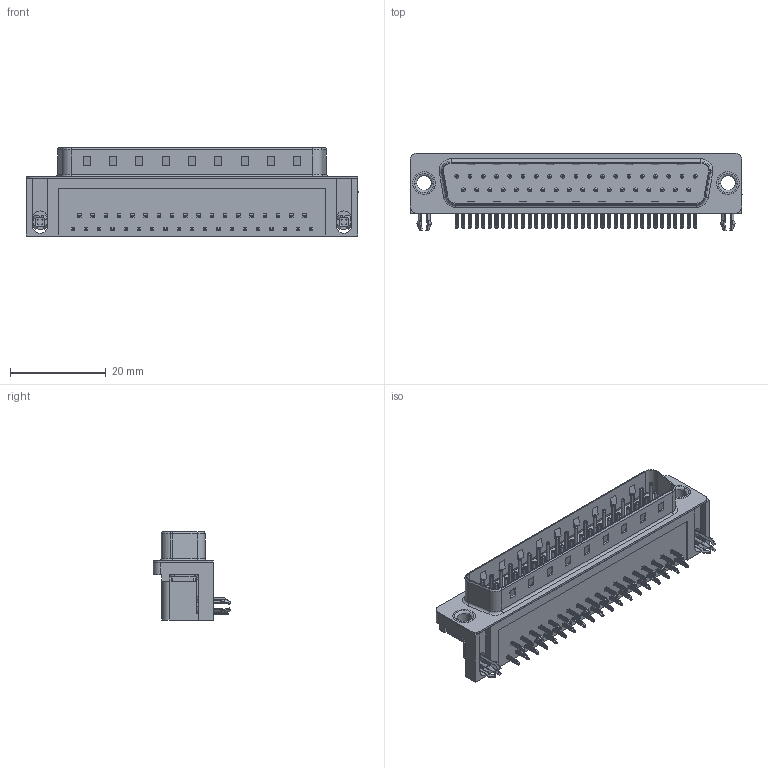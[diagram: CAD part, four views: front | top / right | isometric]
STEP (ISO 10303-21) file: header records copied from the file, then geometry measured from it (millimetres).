
FILE_DESCRIPTION (( 'STEP AP203' ), '1' );
FILE_NAME ('621-037-668-041.STEP', '2019-11-19T11:20:38', ( '' ), ( '' ), 'SwSTEP 2.0', 'SolidWorks 2016', '' );
FILE_SCHEMA (( 'CONFIG_CONTROL_DESIGN' ));
Length unit declared in the file: millimetre
Products named in the file (7): 621 Shell_37 Socket; 621 Thru Hole Rivet; 621 4 Prong Board Lock; 621-037-668-041; 621 Contact Top; 621 Contact Bottom; 621 Housing_37 Socket
Assembly tree (43 placements, depth 2):
  621-037-668-041
    621 Housing_37 Socket
    621 Shell_37 Socket
    621 Contact Bottom  x18
    621 Contact Top  x19
    621 4 Prong Board Lock  x2
    621 Thru Hole Rivet  x2
Bounding box: 69.4 x 16.25 x 18.4 mm (x, y, z)
Volume: 8618.4 mm3; surface area: 10145.5 mm2
Topology: 43 solids, 43 shells, 3279 faces, 8149 edges, 5037 vertices
Faces by surface type: plane 2055, cylinder 903, torus 281, cone 40
Entity records: 26550 total; most frequent: DIRECTION 4375, CARTESIAN_POINT 4304, ORIENTED_EDGE 4140, EDGE_CURVE 2070, LINE 1487, VECTOR 1487, AXIS2_PLACEMENT_3D 1444, VERTEX_POINT 1337
